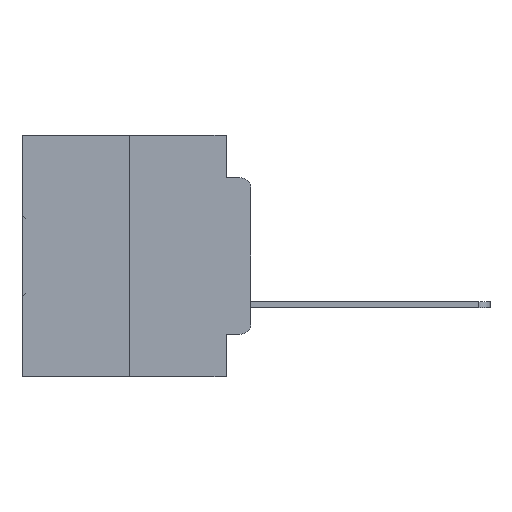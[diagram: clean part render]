
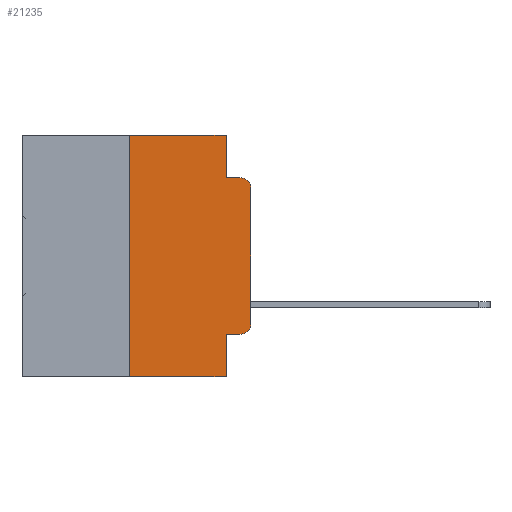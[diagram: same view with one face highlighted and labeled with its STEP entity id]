
A CAD part, left-side view. The second image highlights one B-rep face of the part: STEP entity #21235.
In plain terms, the highlighted planar face has unit normal (-1, 0, 0).
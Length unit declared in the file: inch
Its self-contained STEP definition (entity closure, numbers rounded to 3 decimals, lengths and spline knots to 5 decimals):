
#875 = CARTESIAN_POINT ( 'NONE',  ( 0., 0., -0.1085 ) ) ;
#2744 = CARTESIAN_POINT ( 'NONE',  ( 0., 0., 0. ) ) ;
#3246 = VERTEX_POINT ( 'NONE', #31398 ) ;
#3348 = CIRCLE ( 'NONE', #30798, 0.02 ) ;
#3372 = VECTOR ( 'NONE', #13747, 39.37008 ) ;
#4252 = LINE ( 'NONE', #2744, #3372 ) ;
#4497 = DIRECTION ( 'NONE',  ( 0., 0., -1. ) ) ;
#4618 = VERTEX_POINT ( 'NONE', #32785 ) ;
#5990 = VERTEX_POINT ( 'NONE', #875 ) ;
#6736 = EDGE_CURVE ( 'NONE', #12982, #7586, #25309, .T. ) ;
#7172 = ORIENTED_EDGE ( 'NONE', *, *, #12231, .F. ) ;
#7481 = VERTEX_POINT ( 'NONE', #28950 ) ;
#7586 = VERTEX_POINT ( 'NONE', #31840 ) ;
#8111 = DIRECTION ( 'NONE',  ( 0., 0., -1. ) ) ;
#8282 = ORIENTED_EDGE ( 'NONE', *, *, #30103, .T. ) ;
#8955 = EDGE_LOOP ( 'NONE', ( #25695, #23188, #28047, #7172, #21648, #18664, #16023, #9088, #19275, #8282 ) ) ;
#9088 = ORIENTED_EDGE ( 'NONE', *, *, #6736, .F. ) ;
#9510 = CIRCLE ( 'NONE', #14096, 0.02 ) ;
#9850 = AXIS2_PLACEMENT_3D ( 'NONE', #18703, #23863, #8111 ) ;
#10066 = VECTOR ( 'NONE', #30630, 39.37008 ) ;
#10252 = LINE ( 'NONE', #30238, #23350 ) ;
#10425 = EDGE_CURVE ( 'NONE', #27399, #31060, #10252, .T. ) ;
#10967 = VECTOR ( 'NONE', #33801, 39.37008 ) ;
#11643 = CARTESIAN_POINT ( 'NONE',  ( 0., 0.02, -0.0885 ) ) ;
#12231 = EDGE_CURVE ( 'NONE', #7481, #4618, #19644, .T. ) ;
#12470 = LINE ( 'NONE', #27483, #32484 ) ;
#12672 = LINE ( 'NONE', #31342, #10967 ) ;
#12982 = VERTEX_POINT ( 'NONE', #19610 ) ;
#13747 = DIRECTION ( 'NONE',  ( 0., 0., 1. ) ) ;
#13826 = VERTEX_POINT ( 'NONE', #28594 ) ;
#14096 = AXIS2_PLACEMENT_3D ( 'NONE', #15276, #33052, #17907 ) ;
#14622 = DIRECTION ( 'NONE',  ( 0., -1., 0. ) ) ;
#15105 = DIRECTION ( 'NONE',  ( -1., 0., 0. ) ) ;
#15276 = CARTESIAN_POINT ( 'NONE',  ( 0., 0.02, -0.1085 ) ) ;
#16023 = ORIENTED_EDGE ( 'NONE', *, *, #30329, .T. ) ;
#17370 = CARTESIAN_POINT ( 'NONE',  ( 0., 0.051, 0. ) ) ;
#17907 = DIRECTION ( 'NONE',  ( 0., 0., -1. ) ) ;
#18664 = ORIENTED_EDGE ( 'NONE', *, *, #10425, .F. ) ;
#18703 = CARTESIAN_POINT ( 'NONE',  ( 0., 0.473, 0. ) ) ;
#19258 = EDGE_CURVE ( 'NONE', #4618, #24850, #12470, .T. ) ;
#19275 = ORIENTED_EDGE ( 'NONE', *, *, #31743, .T. ) ;
#19610 = CARTESIAN_POINT ( 'NONE',  ( 0., 0.051, -0.4115 ) ) ;
#19644 = LINE ( 'NONE', #20406, #25643 ) ;
#20406 = CARTESIAN_POINT ( 'NONE',  ( 0., 0.051, 0. ) ) ;
#21000 = EDGE_CURVE ( 'NONE', #5990, #24850, #9510, .T. ) ;
#21235 = ADVANCED_FACE ( 'NONE', ( #24634 ), #26319, .F. ) ;
#21350 = CARTESIAN_POINT ( 'NONE',  ( 0., 0.25, -0.5 ) ) ;
#21648 = ORIENTED_EDGE ( 'NONE', *, *, #32832, .F. ) ;
#22715 = EDGE_CURVE ( 'NONE', #3246, #5990, #4252, .T. ) ;
#23188 = ORIENTED_EDGE ( 'NONE', *, *, #21000, .T. ) ;
#23350 = VECTOR ( 'NONE', #32719, 39.37008 ) ;
#23494 = CARTESIAN_POINT ( 'NONE',  ( 0., 0.473, -0.5 ) ) ;
#23863 = DIRECTION ( 'NONE',  ( 1., 0., 0. ) ) ;
#24634 = FACE_OUTER_BOUND ( 'NONE', #8955, .T. ) ;
#24850 = VERTEX_POINT ( 'NONE', #11643 ) ;
#25110 = DIRECTION ( 'NONE',  ( 0., 0., -1. ) ) ;
#25309 = LINE ( 'NONE', #17370, #31196 ) ;
#25643 = VECTOR ( 'NONE', #4497, 39.37008 ) ;
#25695 = ORIENTED_EDGE ( 'NONE', *, *, #22715, .T. ) ;
#26041 = DIRECTION ( 'NONE',  ( 0., -1., 0. ) ) ;
#26319 = PLANE ( 'NONE',  #9850 ) ;
#27399 = VERTEX_POINT ( 'NONE', #21350 ) ;
#27483 = CARTESIAN_POINT ( 'NONE',  ( 0., 0.051, -0.0885 ) ) ;
#28047 = ORIENTED_EDGE ( 'NONE', *, *, #19258, .F. ) ;
#28175 = CARTESIAN_POINT ( 'NONE',  ( 0., 0.473, 0. ) ) ;
#28594 = CARTESIAN_POINT ( 'NONE',  ( 0., 0.02, -0.4115 ) ) ;
#28950 = CARTESIAN_POINT ( 'NONE',  ( 0., 0.051, 0. ) ) ;
#30103 = EDGE_CURVE ( 'NONE', #13826, #3246, #3348, .T. ) ;
#30238 = CARTESIAN_POINT ( 'NONE',  ( 0., 0.25, 0. ) ) ;
#30329 = EDGE_CURVE ( 'NONE', #27399, #7586, #32369, .T. ) ;
#30432 = CARTESIAN_POINT ( 'NONE',  ( 0., 0.02, -0.3915 ) ) ;
#30630 = DIRECTION ( 'NONE',  ( 0., -1., 0. ) ) ;
#30649 = LINE ( 'NONE', #28175, #10066 ) ;
#30798 = AXIS2_PLACEMENT_3D ( 'NONE', #30432, #15105, #32903 ) ;
#31060 = VERTEX_POINT ( 'NONE', #31166 ) ;
#31166 = CARTESIAN_POINT ( 'NONE',  ( 0., 0.25, 0. ) ) ;
#31196 = VECTOR ( 'NONE', #25110, 39.37008 ) ;
#31342 = CARTESIAN_POINT ( 'NONE',  ( 0., 0.051, -0.4115 ) ) ;
#31398 = CARTESIAN_POINT ( 'NONE',  ( 0., 0., -0.3915 ) ) ;
#31582 = VECTOR ( 'NONE', #26041, 39.37008 ) ;
#31743 = EDGE_CURVE ( 'NONE', #12982, #13826, #12672, .T. ) ;
#31840 = CARTESIAN_POINT ( 'NONE',  ( 0., 0.051, -0.5 ) ) ;
#32369 = LINE ( 'NONE', #23494, #31582 ) ;
#32484 = VECTOR ( 'NONE', #14622, 39.37008 ) ;
#32719 = DIRECTION ( 'NONE',  ( 0., 0., 1. ) ) ;
#32785 = CARTESIAN_POINT ( 'NONE',  ( 0., 0.051, -0.0885 ) ) ;
#32832 = EDGE_CURVE ( 'NONE', #31060, #7481, #30649, .T. ) ;
#32903 = DIRECTION ( 'NONE',  ( 0., 0., -1. ) ) ;
#33052 = DIRECTION ( 'NONE',  ( -1., 0., 0. ) ) ;
#33801 = DIRECTION ( 'NONE',  ( 0., -1., 0. ) ) ;
